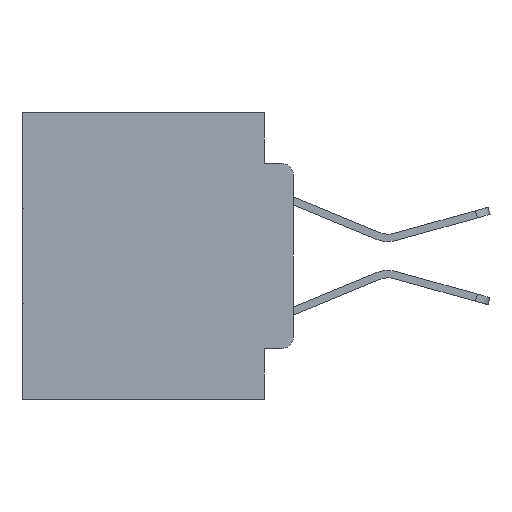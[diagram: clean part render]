
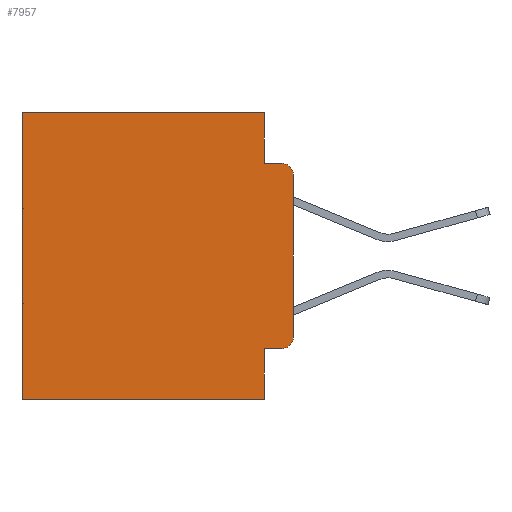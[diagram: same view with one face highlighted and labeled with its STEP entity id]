
A CAD part, left-side view. The second image highlights one B-rep face of the part: STEP entity #7957.
In plain terms, the highlighted planar face has unit normal (-1, 0, 0).
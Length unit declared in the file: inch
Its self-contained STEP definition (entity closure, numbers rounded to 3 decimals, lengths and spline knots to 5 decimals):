
#45 = EDGE_CURVE ( 'NONE', #14723, #26689, #16406, .T. ) ;
#571 = DIRECTION ( 'NONE',  ( 0., 0., -1. ) ) ;
#641 = DIRECTION ( 'NONE',  ( 1., 0., 0. ) ) ;
#1460 = ORIENTED_EDGE ( 'NONE', *, *, #22559, .F. ) ;
#2445 = CARTESIAN_POINT ( 'NONE',  ( 0.298, 0.02, -0.1085 ) ) ;
#2710 = VECTOR ( 'NONE', #28653, 39.37008 ) ;
#2964 = VECTOR ( 'NONE', #29208, 39.37008 ) ;
#3179 = LINE ( 'NONE', #22118, #25752 ) ;
#4710 = CARTESIAN_POINT ( 'NONE',  ( 0.298, 0.02, -0.0885 ) ) ;
#4970 = DIRECTION ( 'NONE',  ( 0., 0., -1. ) ) ;
#5839 = ORIENTED_EDGE ( 'NONE', *, *, #19031, .F. ) ;
#5957 = DIRECTION ( 'NONE',  ( 0., 0., -1. ) ) ;
#6080 = VERTEX_POINT ( 'NONE', #11060 ) ;
#6616 = VERTEX_POINT ( 'NONE', #21290 ) ;
#6781 = VECTOR ( 'NONE', #9201, 39.37008 ) ;
#6848 = CARTESIAN_POINT ( 'NONE',  ( 0.298, 0., -0.5 ) ) ;
#7938 = CARTESIAN_POINT ( 'NONE',  ( 0.298, 0.051, -0.0885 ) ) ;
#7957 = ADVANCED_FACE ( 'NONE', ( #14100 ), #29854, .F. ) ;
#8575 = EDGE_CURVE ( 'NONE', #6616, #12233, #9021, .T. ) ;
#8830 = VERTEX_POINT ( 'NONE', #16520 ) ;
#8961 = DIRECTION ( 'NONE',  ( -1., 0., 0. ) ) ;
#9021 = LINE ( 'NONE', #22485, #15123 ) ;
#9201 = DIRECTION ( 'NONE',  ( 0., 1., 0. ) ) ;
#9917 = AXIS2_PLACEMENT_3D ( 'NONE', #2445, #18870, #4970 ) ;
#10276 = DIRECTION ( 'NONE',  ( 0., -1., 0. ) ) ;
#10291 = ORIENTED_EDGE ( 'NONE', *, *, #45, .F. ) ;
#10574 = CARTESIAN_POINT ( 'NONE',  ( 0.298, 0., 0. ) ) ;
#10849 = CARTESIAN_POINT ( 'NONE',  ( 0.298, 0.051, 0. ) ) ;
#11060 = CARTESIAN_POINT ( 'NONE',  ( 0.298, 0., -0.1085 ) ) ;
#11247 = ORIENTED_EDGE ( 'NONE', *, *, #8575, .T. ) ;
#12090 = ORIENTED_EDGE ( 'NONE', *, *, #21093, .T. ) ;
#12233 = VERTEX_POINT ( 'NONE', #15800 ) ;
#13267 = CARTESIAN_POINT ( 'NONE',  ( 0.298, 0.051, 0. ) ) ;
#14100 = FACE_OUTER_BOUND ( 'NONE', #29671, .T. ) ;
#14120 = AXIS2_PLACEMENT_3D ( 'NONE', #10574, #641, #571 ) ;
#14306 = EDGE_CURVE ( 'NONE', #8830, #24578, #15616, .T. ) ;
#14593 = VECTOR ( 'NONE', #29333, 39.37008 ) ;
#14723 = VERTEX_POINT ( 'NONE', #10849 ) ;
#15123 = VECTOR ( 'NONE', #26775, 39.37008 ) ;
#15514 = LINE ( 'NONE', #26896, #2964 ) ;
#15616 = CIRCLE ( 'NONE', #21544, 0.02 ) ;
#15800 = CARTESIAN_POINT ( 'NONE',  ( 0.298, 0.473, -0.5 ) ) ;
#15832 = EDGE_CURVE ( 'NONE', #24906, #8830, #15870, .T. ) ;
#15870 = LINE ( 'NONE', #24035, #28120 ) ;
#16406 = LINE ( 'NONE', #20877, #28643 ) ;
#16520 = CARTESIAN_POINT ( 'NONE',  ( 0.298, 0.02, -0.4115 ) ) ;
#16928 = ORIENTED_EDGE ( 'NONE', *, *, #14306, .T. ) ;
#17841 = CIRCLE ( 'NONE', #9917, 0.02 ) ;
#18534 = CARTESIAN_POINT ( 'NONE',  ( 0.298, 0.051, -0.4115 ) ) ;
#18870 = DIRECTION ( 'NONE',  ( -1., 0., 0. ) ) ;
#19031 = EDGE_CURVE ( 'NONE', #27872, #12233, #25150, .T. ) ;
#19671 = CARTESIAN_POINT ( 'NONE',  ( 0.298, 0., -0.3915 ) ) ;
#20669 = LINE ( 'NONE', #13267, #14593 ) ;
#20746 = EDGE_CURVE ( 'NONE', #6080, #24578, #3179, .T. ) ;
#20877 = CARTESIAN_POINT ( 'NONE',  ( 0.298, 0.051, 0. ) ) ;
#21093 = EDGE_CURVE ( 'NONE', #6080, #24962, #17841, .T. ) ;
#21286 = CARTESIAN_POINT ( 'NONE',  ( 0.298, 0.051, -0.5 ) ) ;
#21290 = CARTESIAN_POINT ( 'NONE',  ( 0.298, 0.473, 0. ) ) ;
#21450 = EDGE_CURVE ( 'NONE', #24906, #27872, #20669, .T. ) ;
#21544 = AXIS2_PLACEMENT_3D ( 'NONE', #22712, #8961, #25027 ) ;
#22118 = CARTESIAN_POINT ( 'NONE',  ( 0.298, 0., 0. ) ) ;
#22485 = CARTESIAN_POINT ( 'NONE',  ( 0.298, 0.473, 0. ) ) ;
#22559 = EDGE_CURVE ( 'NONE', #26689, #24962, #27512, .T. ) ;
#22712 = CARTESIAN_POINT ( 'NONE',  ( 0.298, 0.02, -0.3915 ) ) ;
#22893 = DIRECTION ( 'NONE',  ( 0., 0., -1. ) ) ;
#24035 = CARTESIAN_POINT ( 'NONE',  ( 0.298, 0.051, -0.4115 ) ) ;
#24578 = VERTEX_POINT ( 'NONE', #19671 ) ;
#24702 = ORIENTED_EDGE ( 'NONE', *, *, #21450, .F. ) ;
#24906 = VERTEX_POINT ( 'NONE', #18534 ) ;
#24962 = VERTEX_POINT ( 'NONE', #4710 ) ;
#25027 = DIRECTION ( 'NONE',  ( 0., 0., -1. ) ) ;
#25150 = LINE ( 'NONE', #6848, #6781 ) ;
#25561 = ORIENTED_EDGE ( 'NONE', *, *, #15832, .T. ) ;
#25752 = VECTOR ( 'NONE', #5957, 39.37008 ) ;
#25910 = ORIENTED_EDGE ( 'NONE', *, *, #20746, .F. ) ;
#26689 = VERTEX_POINT ( 'NONE', #28707 ) ;
#26775 = DIRECTION ( 'NONE',  ( 0., 0., -1. ) ) ;
#26803 = EDGE_CURVE ( 'NONE', #14723, #6616, #15514, .T. ) ;
#26896 = CARTESIAN_POINT ( 'NONE',  ( 0.298, 0., 0. ) ) ;
#27132 = ORIENTED_EDGE ( 'NONE', *, *, #26803, .T. ) ;
#27512 = LINE ( 'NONE', #7938, #2710 ) ;
#27872 = VERTEX_POINT ( 'NONE', #21286 ) ;
#28120 = VECTOR ( 'NONE', #10276, 39.37008 ) ;
#28643 = VECTOR ( 'NONE', #22893, 39.37008 ) ;
#28653 = DIRECTION ( 'NONE',  ( 0., -1., 0. ) ) ;
#28707 = CARTESIAN_POINT ( 'NONE',  ( 0.298, 0.051, -0.0885 ) ) ;
#29208 = DIRECTION ( 'NONE',  ( 0., 1., 0. ) ) ;
#29333 = DIRECTION ( 'NONE',  ( 0., 0., -1. ) ) ;
#29671 = EDGE_LOOP ( 'NONE', ( #25910, #12090, #1460, #10291, #27132, #11247, #5839, #24702, #25561, #16928 ) ) ;
#29854 = PLANE ( 'NONE',  #14120 ) ;
